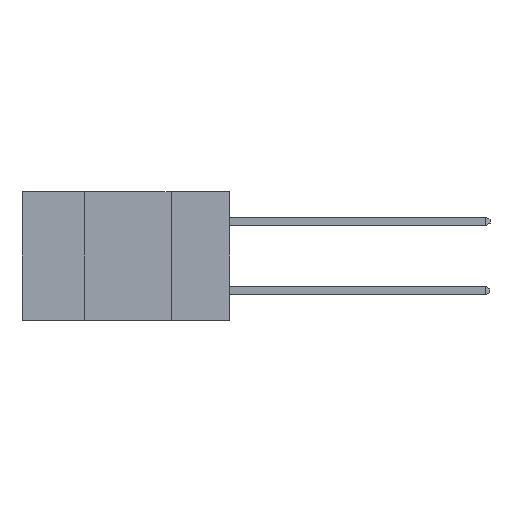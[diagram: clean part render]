
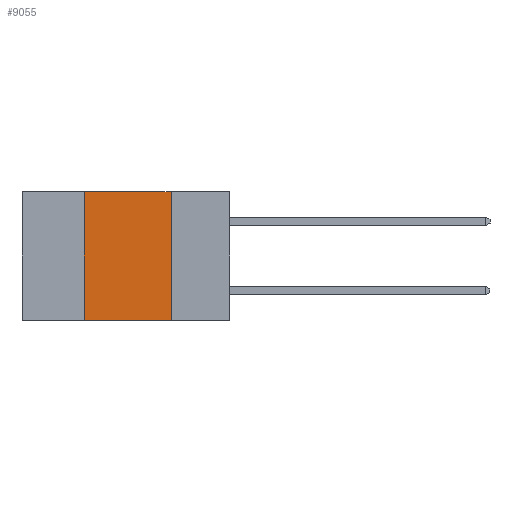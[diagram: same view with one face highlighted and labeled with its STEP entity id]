
A CAD part, left-side view. The second image highlights one B-rep face of the part: STEP entity #9055.
In plain terms, the highlighted planar face has unit normal (-1, 0, 0).
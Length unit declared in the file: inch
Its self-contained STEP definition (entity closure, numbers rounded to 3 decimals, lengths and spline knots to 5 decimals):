
#318 = VERTEX_POINT ( 'NONE', #9684 ) ;
#726 = LINE ( 'NONE', #3363, #6040 ) ;
#1146 = EDGE_CURVE ( 'NONE', #9953, #318, #5141, .T. ) ;
#1263 = DIRECTION ( 'NONE',  ( 1., 0., 0. ) ) ;
#1469 = CARTESIAN_POINT ( 'NONE',  ( 0., 0.6, 0. ) ) ;
#1879 = VECTOR ( 'NONE', #6439, 39.37008 ) ;
#3034 = DIRECTION ( 'NONE',  ( 0., 0., -1. ) ) ;
#3176 = LINE ( 'NONE', #8954, #8140 ) ;
#3227 = CARTESIAN_POINT ( 'NONE',  ( 0., 0.6, 0. ) ) ;
#3228 = CARTESIAN_POINT ( 'NONE',  ( 0., 0.17, -0.37 ) ) ;
#3363 = CARTESIAN_POINT ( 'NONE',  ( 0., 0.6, -0.37 ) ) ;
#4418 = VERTEX_POINT ( 'NONE', #3228 ) ;
#4497 = VECTOR ( 'NONE', #10123, 39.37008 ) ;
#4586 = EDGE_LOOP ( 'NONE', ( #11578, #9671, #12119, #9985 ) ) ;
#5141 = LINE ( 'NONE', #9464, #4497 ) ;
#6040 = VECTOR ( 'NONE', #10261, 39.37008 ) ;
#6195 = CARTESIAN_POINT ( 'NONE',  ( 0., 0.17, 0. ) ) ;
#6439 = DIRECTION ( 'NONE',  ( 0., -1., 0. ) ) ;
#6525 = EDGE_CURVE ( 'NONE', #318, #9016, #9787, .T. ) ;
#7241 = PLANE ( 'NONE',  #7610 ) ;
#7610 = AXIS2_PLACEMENT_3D ( 'NONE', #3227, #1263, #8205 ) ;
#8140 = VECTOR ( 'NONE', #3034, 39.37008 ) ;
#8205 = DIRECTION ( 'NONE',  ( 0., 0., -1. ) ) ;
#8954 = CARTESIAN_POINT ( 'NONE',  ( 0., 0.17, 0. ) ) ;
#9016 = VERTEX_POINT ( 'NONE', #6195 ) ;
#9055 = ADVANCED_FACE ( 'NONE', ( #11749 ), #7241, .F. ) ;
#9110 = EDGE_CURVE ( 'NONE', #9953, #4418, #726, .T. ) ;
#9464 = CARTESIAN_POINT ( 'NONE',  ( 0., 0.42, 0. ) ) ;
#9671 = ORIENTED_EDGE ( 'NONE', *, *, #6525, .F. ) ;
#9684 = CARTESIAN_POINT ( 'NONE',  ( 0., 0.42, 0. ) ) ;
#9787 = LINE ( 'NONE', #1469, #1879 ) ;
#9953 = VERTEX_POINT ( 'NONE', #10445 ) ;
#9985 = ORIENTED_EDGE ( 'NONE', *, *, #9110, .T. ) ;
#10123 = DIRECTION ( 'NONE',  ( 0., 0., 1. ) ) ;
#10261 = DIRECTION ( 'NONE',  ( 0., -1., 0. ) ) ;
#10445 = CARTESIAN_POINT ( 'NONE',  ( 0., 0.42, -0.37 ) ) ;
#11578 = ORIENTED_EDGE ( 'NONE', *, *, #11657, .F. ) ;
#11657 = EDGE_CURVE ( 'NONE', #9016, #4418, #3176, .T. ) ;
#11749 = FACE_OUTER_BOUND ( 'NONE', #4586, .T. ) ;
#12119 = ORIENTED_EDGE ( 'NONE', *, *, #1146, .F. ) ;
